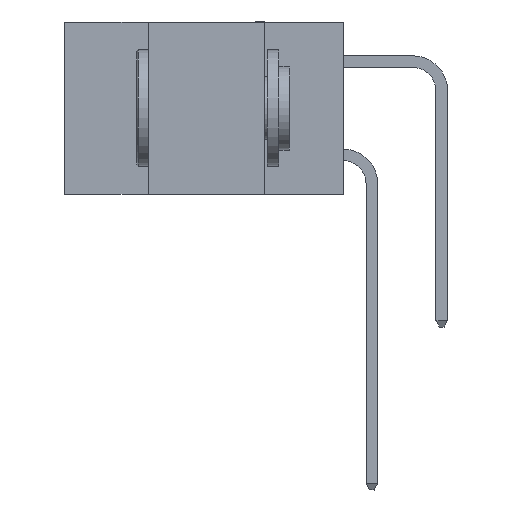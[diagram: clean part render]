
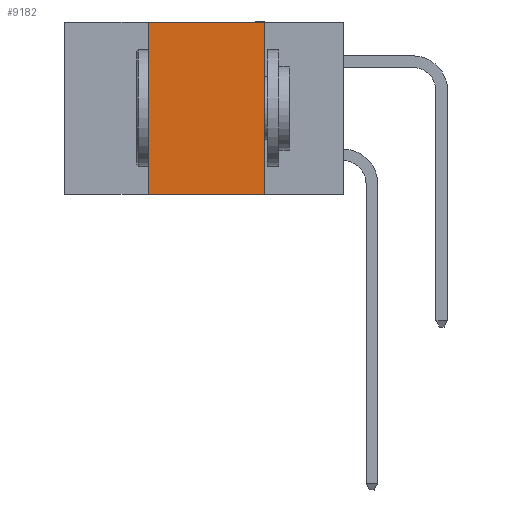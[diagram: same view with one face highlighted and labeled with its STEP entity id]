
A CAD part, left-side view. The second image highlights one B-rep face of the part: STEP entity #9182.
In plain terms, the highlighted planar face has unit normal (-1, 0, 0).
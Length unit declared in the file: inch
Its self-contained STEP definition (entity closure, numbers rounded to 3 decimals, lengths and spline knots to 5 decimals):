
#147 = VERTEX_POINT ( 'NONE', #11840 ) ;
#423 = VECTOR ( 'NONE', #18808, 39.37008 ) ;
#592 = ORIENTED_EDGE ( 'NONE', *, *, #14672, .F. ) ;
#2651 = CARTESIAN_POINT ( 'NONE',  ( 0., 0.6, -0.37 ) ) ;
#2835 = LINE ( 'NONE', #22224, #7733 ) ;
#2917 = AXIS2_PLACEMENT_3D ( 'NONE', #12185, #23412, #25658 ) ;
#3452 = PLANE ( 'NONE',  #2917 ) ;
#4333 = ORIENTED_EDGE ( 'NONE', *, *, #8599, .T. ) ;
#5902 = EDGE_LOOP ( 'NONE', ( #12134, #592, #20364, #4333 ) ) ;
#7733 = VECTOR ( 'NONE', #17789, 39.37008 ) ;
#7798 = CARTESIAN_POINT ( 'NONE',  ( 0., 0.42, -0.37 ) ) ;
#8599 = EDGE_CURVE ( 'NONE', #22903, #11291, #28348, .T. ) ;
#9182 = ADVANCED_FACE ( 'NONE', ( #18242 ), #3452, .F. ) ;
#11291 = VERTEX_POINT ( 'NONE', #19993 ) ;
#11533 = EDGE_CURVE ( 'NONE', #22903, #15312, #21075, .T. ) ;
#11840 = CARTESIAN_POINT ( 'NONE',  ( 0., 0.17, 0. ) ) ;
#12134 = ORIENTED_EDGE ( 'NONE', *, *, #14271, .F. ) ;
#12185 = CARTESIAN_POINT ( 'NONE',  ( 0., 0.6, 0. ) ) ;
#13764 = VECTOR ( 'NONE', #27166, 39.37008 ) ;
#14271 = EDGE_CURVE ( 'NONE', #147, #11291, #2835, .T. ) ;
#14672 = EDGE_CURVE ( 'NONE', #15312, #147, #22948, .T. ) ;
#15312 = VERTEX_POINT ( 'NONE', #20113 ) ;
#17789 = DIRECTION ( 'NONE',  ( 0., 0., -1. ) ) ;
#18242 = FACE_OUTER_BOUND ( 'NONE', #5902, .T. ) ;
#18808 = DIRECTION ( 'NONE',  ( 0., -1., 0. ) ) ;
#19993 = CARTESIAN_POINT ( 'NONE',  ( 0., 0.17, -0.37 ) ) ;
#20113 = CARTESIAN_POINT ( 'NONE',  ( 0., 0.42, 0. ) ) ;
#20364 = ORIENTED_EDGE ( 'NONE', *, *, #11533, .F. ) ;
#21075 = LINE ( 'NONE', #22663, #26604 ) ;
#22224 = CARTESIAN_POINT ( 'NONE',  ( 0., 0.17, 0. ) ) ;
#22663 = CARTESIAN_POINT ( 'NONE',  ( 0., 0.42, 0. ) ) ;
#22903 = VERTEX_POINT ( 'NONE', #7798 ) ;
#22948 = LINE ( 'NONE', #25397, #423 ) ;
#23412 = DIRECTION ( 'NONE',  ( 1., 0., 0. ) ) ;
#25397 = CARTESIAN_POINT ( 'NONE',  ( 0., 0.6, 0. ) ) ;
#25658 = DIRECTION ( 'NONE',  ( 0., 0., -1. ) ) ;
#26604 = VECTOR ( 'NONE', #27221, 39.37008 ) ;
#27166 = DIRECTION ( 'NONE',  ( 0., -1., 0. ) ) ;
#27221 = DIRECTION ( 'NONE',  ( 0., 0., 1. ) ) ;
#28348 = LINE ( 'NONE', #2651, #13764 ) ;
